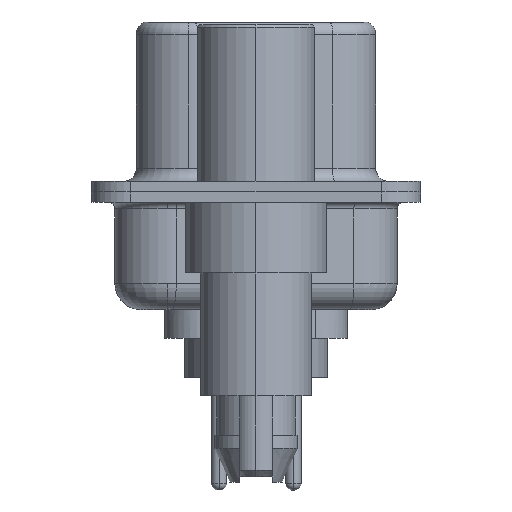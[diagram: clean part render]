
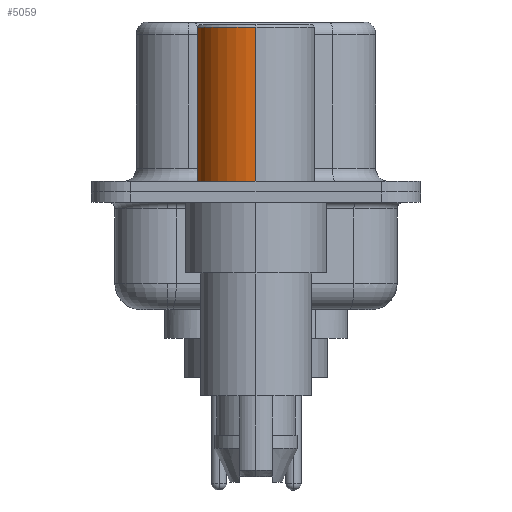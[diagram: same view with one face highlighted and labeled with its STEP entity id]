
A CAD part, left-side view. The second image highlights one B-rep face of the part: STEP entity #5059.
In plain terms, the highlighted cylindrical face has radius 2.25 mm (diameter 4.5 mm), a partial arc.
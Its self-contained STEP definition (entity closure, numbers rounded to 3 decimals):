
#514 = VERTEX_POINT ( 'NONE', #3422 ) ;
#1621 = VECTOR ( 'NONE', #4345, 1000. ) ;
#2479 = DIRECTION ( 'NONE',  ( 1., 0., 0. ) ) ;
#2638 = EDGE_CURVE ( 'NONE', #6403, #16043, #8812, .T. ) ;
#3157 = DIRECTION ( 'NONE',  ( 0., 0., 1. ) ) ;
#3422 = CARTESIAN_POINT ( 'NONE',  ( 2.25, 0., 6.3 ) ) ;
#3505 = VERTEX_POINT ( 'NONE', #16414 ) ;
#3994 = LINE ( 'NONE', #6857, #7359 ) ;
#4345 = DIRECTION ( 'NONE',  ( 0., 0., 1. ) ) ;
#4982 = AXIS2_PLACEMENT_3D ( 'NONE', #12349, #3157, #18468 ) ;
#5059 = ADVANCED_FACE ( 'NONE', ( #16199 ), #15971, .T. ) ;
#5389 = EDGE_CURVE ( 'NONE', #16043, #3505, #7832, .T. ) ;
#6403 = VERTEX_POINT ( 'NONE', #8863 ) ;
#6551 = AXIS2_PLACEMENT_3D ( 'NONE', #14166, #18655, #8096 ) ;
#6857 = CARTESIAN_POINT ( 'NONE',  ( 2.25, 0., 0.581 ) ) ;
#7359 = VECTOR ( 'NONE', #17533, 1000. ) ;
#7392 = CIRCLE ( 'NONE', #6551, 2.25 ) ;
#7832 = LINE ( 'NONE', #19689, #1621 ) ;
#8096 = DIRECTION ( 'NONE',  ( 1., 0., 0. ) ) ;
#8436 = DIRECTION ( 'NONE',  ( 0., 0., 1. ) ) ;
#8812 = CIRCLE ( 'NONE', #4982, 2.25 ) ;
#8863 = CARTESIAN_POINT ( 'NONE',  ( 2.25, 0., 0.4 ) ) ;
#9412 = ORIENTED_EDGE ( 'NONE', *, *, #2638, .T. ) ;
#10032 = AXIS2_PLACEMENT_3D ( 'NONE', #11721, #8436, #2479 ) ;
#11511 = EDGE_LOOP ( 'NONE', ( #9412, #12708, #12541, #13274 ) ) ;
#11721 = CARTESIAN_POINT ( 'NONE',  ( 0., 0., 0.581 ) ) ;
#12349 = CARTESIAN_POINT ( 'NONE',  ( 0., 0., 0.4 ) ) ;
#12541 = ORIENTED_EDGE ( 'NONE', *, *, #13704, .F. ) ;
#12708 = ORIENTED_EDGE ( 'NONE', *, *, #5389, .T. ) ;
#13274 = ORIENTED_EDGE ( 'NONE', *, *, #14513, .F. ) ;
#13704 = EDGE_CURVE ( 'NONE', #514, #3505, #7392, .T. ) ;
#14166 = CARTESIAN_POINT ( 'NONE',  ( 0., 0., 6.3 ) ) ;
#14513 = EDGE_CURVE ( 'NONE', #6403, #514, #3994, .T. ) ;
#15971 = CYLINDRICAL_SURFACE ( 'NONE', #10032, 2.25 ) ;
#16043 = VERTEX_POINT ( 'NONE', #16928 ) ;
#16199 = FACE_OUTER_BOUND ( 'NONE', #11511, .T. ) ;
#16414 = CARTESIAN_POINT ( 'NONE',  ( -2.25, 0., 6.3 ) ) ;
#16928 = CARTESIAN_POINT ( 'NONE',  ( -2.25, 0., 0.4 ) ) ;
#17533 = DIRECTION ( 'NONE',  ( 0., 0., 1. ) ) ;
#18468 = DIRECTION ( 'NONE',  ( 1., 0., 0. ) ) ;
#18655 = DIRECTION ( 'NONE',  ( 0., 0., 1. ) ) ;
#19689 = CARTESIAN_POINT ( 'NONE',  ( -2.25, 0., 0.581 ) ) ;
